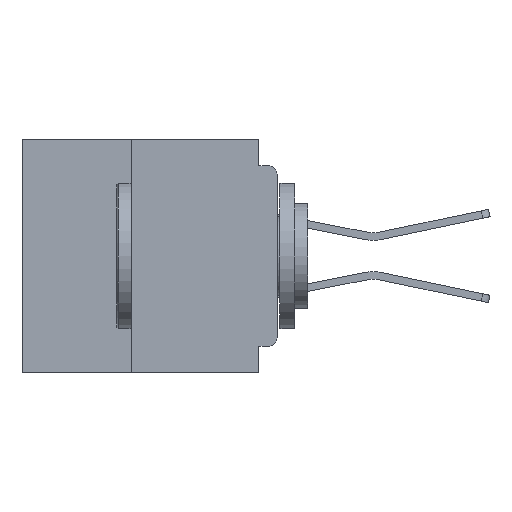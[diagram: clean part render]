
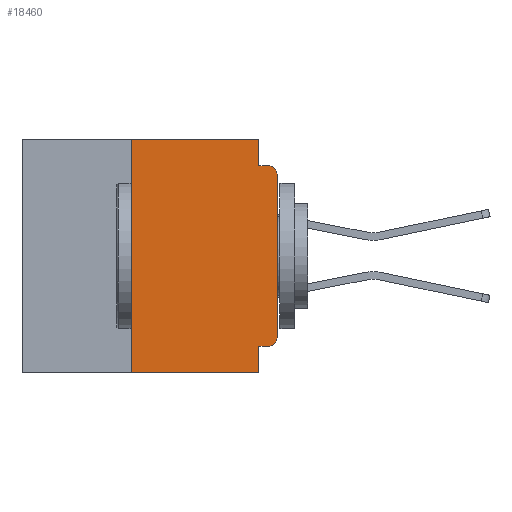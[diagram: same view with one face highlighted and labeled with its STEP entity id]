
A CAD part, left-side view. The second image highlights one B-rep face of the part: STEP entity #18460.
In plain terms, the highlighted planar face has unit normal (-1, 0, 0).
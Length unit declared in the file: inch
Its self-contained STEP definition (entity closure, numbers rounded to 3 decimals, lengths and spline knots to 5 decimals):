
#352 = CARTESIAN_POINT ( 'NONE',  ( 0., 0.015, -0.045 ) ) ;
#1569 = CARTESIAN_POINT ( 'NONE',  ( 0., 0., -0.34 ) ) ;
#1691 = ORIENTED_EDGE ( 'NONE', *, *, #32083, .F. ) ;
#2321 = VECTOR ( 'NONE', #39974, 39.37008 ) ;
#2457 = DIRECTION ( 'NONE',  ( 0., -1., 0. ) ) ;
#2688 = VERTEX_POINT ( 'NONE', #352 ) ;
#2750 = ORIENTED_EDGE ( 'NONE', *, *, #37562, .T. ) ;
#3343 = LINE ( 'NONE', #33379, #2321 ) ;
#3635 = DIRECTION ( 'NONE',  ( 0., 0., 1. ) ) ;
#3967 = LINE ( 'NONE', #36145, #28572 ) ;
#4664 = CARTESIAN_POINT ( 'NONE',  ( 0., 0.031, -0.4 ) ) ;
#5082 = EDGE_CURVE ( 'NONE', #31980, #24599, #36613, .T. ) ;
#6034 = FACE_OUTER_BOUND ( 'NONE', #6775, .T. ) ;
#6503 = CARTESIAN_POINT ( 'NONE',  ( 0., 0., -0.06 ) ) ;
#6775 = EDGE_LOOP ( 'NONE', ( #6902, #42538, #18939, #28890, #32070, #34170, #43087, #1691, #19490, #2750 ) ) ;
#6902 = ORIENTED_EDGE ( 'NONE', *, *, #26240, .T. ) ;
#8139 = DIRECTION ( 'NONE',  ( 0., -1., 0. ) ) ;
#8753 = AXIS2_PLACEMENT_3D ( 'NONE', #14141, #37542, #17448 ) ;
#10066 = CIRCLE ( 'NONE', #24642, 0.015 ) ;
#10403 = CARTESIAN_POINT ( 'NONE',  ( 0., 0.015, -0.06 ) ) ;
#10521 = VECTOR ( 'NONE', #3635, 39.37008 ) ;
#10823 = VERTEX_POINT ( 'NONE', #37865 ) ;
#11541 = CARTESIAN_POINT ( 'NONE',  ( 0., 0.437, -0.4 ) ) ;
#12669 = DIRECTION ( 'NONE',  ( 0., 0., 1. ) ) ;
#13631 = CARTESIAN_POINT ( 'NONE',  ( 0., 0., 0. ) ) ;
#13756 = DIRECTION ( 'NONE',  ( 0., 0., -1. ) ) ;
#13858 = CIRCLE ( 'NONE', #8753, 0.015 ) ;
#14141 = CARTESIAN_POINT ( 'NONE',  ( 0., 0.015, -0.34 ) ) ;
#14477 = EDGE_CURVE ( 'NONE', #10823, #2688, #25676, .T. ) ;
#16680 = LINE ( 'NONE', #25905, #25587 ) ;
#17059 = EDGE_CURVE ( 'NONE', #31980, #17344, #26012, .T. ) ;
#17344 = VERTEX_POINT ( 'NONE', #34107 ) ;
#17448 = DIRECTION ( 'NONE',  ( 0., 0., -1. ) ) ;
#17837 = CARTESIAN_POINT ( 'NONE',  ( 0., 0.437, 0. ) ) ;
#18157 = CARTESIAN_POINT ( 'NONE',  ( 0., 0.015, -0.355 ) ) ;
#18460 = ADVANCED_FACE ( 'NONE', ( #6034 ), #34568, .F. ) ;
#18939 = ORIENTED_EDGE ( 'NONE', *, *, #14477, .F. ) ;
#19180 = DIRECTION ( 'NONE',  ( 0., 0., -1. ) ) ;
#19382 = LINE ( 'NONE', #13631, #10521 ) ;
#19490 = ORIENTED_EDGE ( 'NONE', *, *, #30457, .F. ) ;
#21213 = DIRECTION ( 'NONE',  ( 0., 0., -1. ) ) ;
#21751 = VECTOR ( 'NONE', #32670, 39.37008 ) ;
#22126 = VERTEX_POINT ( 'NONE', #36114 ) ;
#24599 = VERTEX_POINT ( 'NONE', #4664 ) ;
#24642 = AXIS2_PLACEMENT_3D ( 'NONE', #10403, #33786, #13756 ) ;
#25268 = AXIS2_PLACEMENT_3D ( 'NONE', #17837, #41306, #21213 ) ;
#25587 = VECTOR ( 'NONE', #19180, 39.37008 ) ;
#25676 = LINE ( 'NONE', #32471, #42465 ) ;
#25905 = CARTESIAN_POINT ( 'NONE',  ( 0., 0.031, -0.4 ) ) ;
#26012 = LINE ( 'NONE', #29281, #42819 ) ;
#26240 = EDGE_CURVE ( 'NONE', #39912, #38834, #19382, .T. ) ;
#28183 = VERTEX_POINT ( 'NONE', #28784 ) ;
#28572 = VECTOR ( 'NONE', #39519, 39.37008 ) ;
#28784 = CARTESIAN_POINT ( 'NONE',  ( 0., 0.031, -0.355 ) ) ;
#28890 = ORIENTED_EDGE ( 'NONE', *, *, #34408, .F. ) ;
#29281 = CARTESIAN_POINT ( 'NONE',  ( 0., 0.25, -0.4 ) ) ;
#30457 = EDGE_CURVE ( 'NONE', #35853, #28183, #3343, .T. ) ;
#31980 = VERTEX_POINT ( 'NONE', #42209 ) ;
#32070 = ORIENTED_EDGE ( 'NONE', *, *, #33774, .F. ) ;
#32083 = EDGE_CURVE ( 'NONE', #28183, #24599, #16680, .T. ) ;
#32471 = CARTESIAN_POINT ( 'NONE',  ( 0., 0., -0.045 ) ) ;
#32670 = DIRECTION ( 'NONE',  ( 0., -1., 0. ) ) ;
#33379 = CARTESIAN_POINT ( 'NONE',  ( 0., 0., -0.355 ) ) ;
#33774 = EDGE_CURVE ( 'NONE', #17344, #22126, #39620, .T. ) ;
#33786 = DIRECTION ( 'NONE',  ( -1., 0., 0. ) ) ;
#34107 = CARTESIAN_POINT ( 'NONE',  ( 0., 0.25, 0. ) ) ;
#34170 = ORIENTED_EDGE ( 'NONE', *, *, #17059, .F. ) ;
#34408 = EDGE_CURVE ( 'NONE', #22126, #10823, #3967, .T. ) ;
#34568 = PLANE ( 'NONE',  #25268 ) ;
#35853 = VERTEX_POINT ( 'NONE', #18157 ) ;
#36114 = CARTESIAN_POINT ( 'NONE',  ( 0., 0.031, 0. ) ) ;
#36145 = CARTESIAN_POINT ( 'NONE',  ( 0., 0.031, 0. ) ) ;
#36613 = LINE ( 'NONE', #11541, #43403 ) ;
#36864 = EDGE_CURVE ( 'NONE', #38834, #2688, #10066, .T. ) ;
#37542 = DIRECTION ( 'NONE',  ( -1., 0., 0. ) ) ;
#37562 = EDGE_CURVE ( 'NONE', #35853, #39912, #13858, .T. ) ;
#37865 = CARTESIAN_POINT ( 'NONE',  ( 0., 0.031, -0.045 ) ) ;
#38834 = VERTEX_POINT ( 'NONE', #6503 ) ;
#39519 = DIRECTION ( 'NONE',  ( 0., 0., -1. ) ) ;
#39620 = LINE ( 'NONE', #42488, #21751 ) ;
#39912 = VERTEX_POINT ( 'NONE', #1569 ) ;
#39974 = DIRECTION ( 'NONE',  ( 0., 1., 0. ) ) ;
#41306 = DIRECTION ( 'NONE',  ( 1., 0., 0. ) ) ;
#42209 = CARTESIAN_POINT ( 'NONE',  ( 0., 0.25, -0.4 ) ) ;
#42465 = VECTOR ( 'NONE', #2457, 39.37008 ) ;
#42488 = CARTESIAN_POINT ( 'NONE',  ( 0., 0.437, 0. ) ) ;
#42538 = ORIENTED_EDGE ( 'NONE', *, *, #36864, .T. ) ;
#42819 = VECTOR ( 'NONE', #12669, 39.37008 ) ;
#43087 = ORIENTED_EDGE ( 'NONE', *, *, #5082, .T. ) ;
#43403 = VECTOR ( 'NONE', #8139, 39.37008 ) ;
